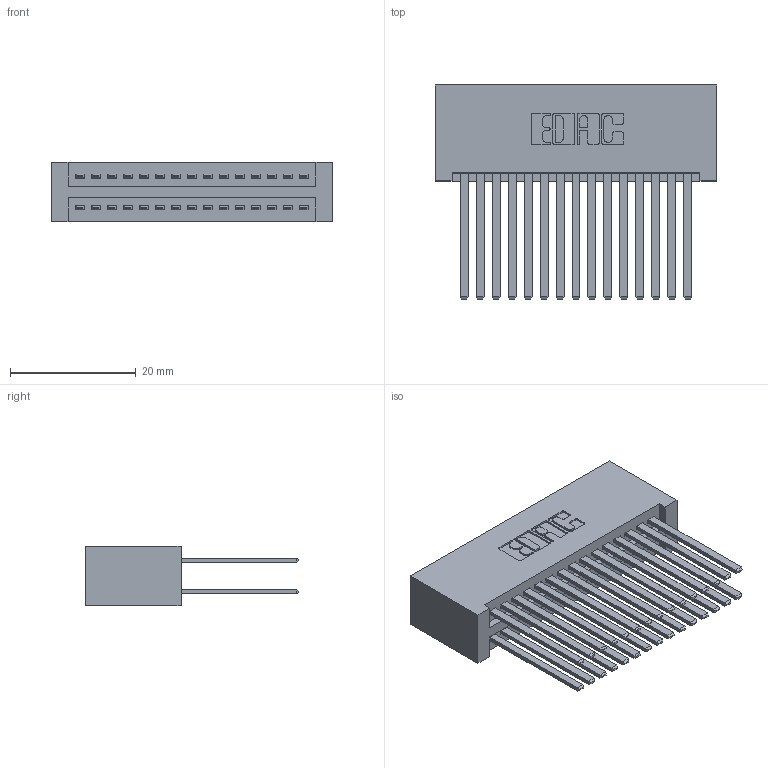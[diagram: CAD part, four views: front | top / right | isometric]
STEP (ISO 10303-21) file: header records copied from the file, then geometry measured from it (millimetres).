
FILE_DESCRIPTION (( 'STEP AP203' ), '1' );
FILE_NAME ('395-030-544-201.STEP', '2019-10-17T14:35:17', ( '' ), ( '' ), 'SwSTEP 2.0', 'SolidWorks 2016', '' );
FILE_SCHEMA (( 'CONFIG_CONTROL_DESIGN' ));
Length unit declared in the file: inch
Products named in the file (3): 345 Part_No Mounting Lugs; 345-292-001_345-293-144; 395-030-544-201
Assembly tree (31 placements, depth 2):
  395-030-544-201
    345 Part_No Mounting Lugs
    345-292-001_345-293-144  x30
Bounding box: 44.7 x 33.96 x 9.4 mm (x, y, z)
Volume: 5128.4 mm3; surface area: 8593.6 mm2
Topology: 31 solids, 31 shells, 1438 faces, 4247 edges, 2790 vertices
Faces by surface type: plane 946, cylinder 492
Entity records: 14943 total; most frequent: CARTESIAN_POINT 2528, ORIENTED_EDGE 2462, DIRECTION 2255, EDGE_CURVE 1231, VECTOR 1051, LINE 1051, VERTEX_POINT 818, AXIS2_PLACEMENT_3D 602
